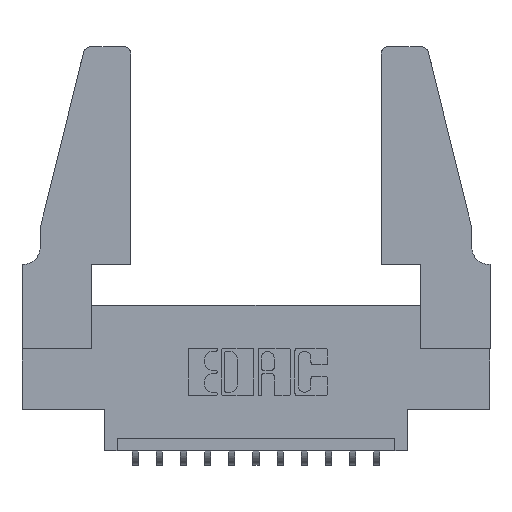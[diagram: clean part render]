
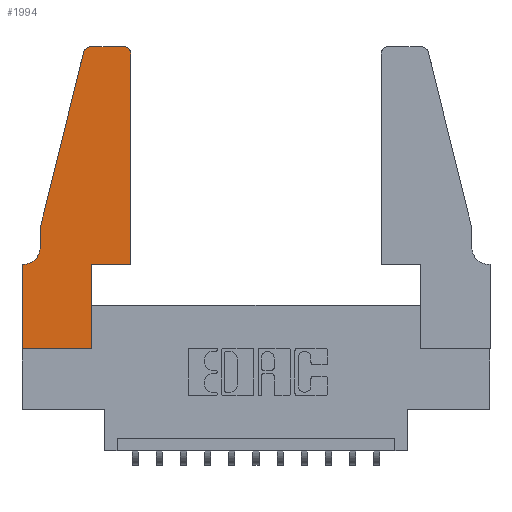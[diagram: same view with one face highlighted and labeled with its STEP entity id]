
A CAD part, top view. The second image highlights one B-rep face of the part: STEP entity #1994.
In plain terms, the highlighted planar face has unit normal (0, 0, 1).
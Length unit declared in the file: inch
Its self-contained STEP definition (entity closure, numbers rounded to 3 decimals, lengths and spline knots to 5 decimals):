
#477 = CIRCLE ( 'NONE', #2030, 0.03 ) ;
#761 = EDGE_CURVE ( 'NONE', #6258, #11032, #4310, .T. ) ;
#1099 = CARTESIAN_POINT ( 'NONE',  ( 0., 0.35, 0.37 ) ) ;
#1384 = DIRECTION ( 'NONE',  ( -1., 0., 0. ) ) ;
#1393 = VERTEX_POINT ( 'NONE', #7860 ) ;
#1628 = ORIENTED_EDGE ( 'NONE', *, *, #12560, .T. ) ;
#1816 = EDGE_CURVE ( 'NONE', #11215, #7430, #12489, .T. ) ;
#1901 = CARTESIAN_POINT ( 'NONE',  ( 0.4505, 0.35, 0.37 ) ) ;
#1978 = CARTESIAN_POINT ( 'NONE',  ( 0., 0.35, 0.37 ) ) ;
#1994 = ADVANCED_FACE ( 'NONE', ( #3218 ), #10353, .T. ) ;
#2030 = AXIS2_PLACEMENT_3D ( 'NONE', #9277, #3064, #12855 ) ;
#2187 = DIRECTION ( 'NONE',  ( 0., 0., 1. ) ) ;
#2191 = LINE ( 'NONE', #6546, #3615 ) ;
#2400 = CIRCLE ( 'NONE', #6021, 0.03 ) ;
#2414 = DIRECTION ( 'NONE',  ( 1., 0., 0. ) ) ;
#2422 = CARTESIAN_POINT ( 'NONE',  ( 0.0755, 0.42, 0.37 ) ) ;
#2580 = AXIS2_PLACEMENT_3D ( 'NONE', #4893, #10802, #13399 ) ;
#2738 = VERTEX_POINT ( 'NONE', #6799 ) ;
#2871 = CARTESIAN_POINT ( 'NONE',  ( 0.4205, 1.22, 0.37 ) ) ;
#3064 = DIRECTION ( 'NONE',  ( 0., 0., 1. ) ) ;
#3211 = VECTOR ( 'NONE', #9540, 39.37008 ) ;
#3218 = FACE_OUTER_BOUND ( 'NONE', #13090, .T. ) ;
#3220 = CARTESIAN_POINT ( 'NONE',  ( 0.284, 1.25, 0.37 ) ) ;
#3224 = VERTEX_POINT ( 'NONE', #11091 ) ;
#3413 = CARTESIAN_POINT ( 'NONE',  ( 0.0055, 0.35, 0.37 ) ) ;
#3503 = CIRCLE ( 'NONE', #2580, 0.07 ) ;
#3611 = CARTESIAN_POINT ( 'NONE',  ( 0.2865, 0.35, 0.37 ) ) ;
#3615 = VECTOR ( 'NONE', #13312, 39.37008 ) ;
#3665 = DIRECTION ( 'NONE',  ( 0., 1., 0. ) ) ;
#3710 = LINE ( 'NONE', #7285, #3211 ) ;
#3768 = EDGE_CURVE ( 'NONE', #5667, #11215, #3503, .T. ) ;
#3890 = ORIENTED_EDGE ( 'NONE', *, *, #11696, .T. ) ;
#4013 = CARTESIAN_POINT ( 'NONE',  ( 0.4505, 0.35, 0.37 ) ) ;
#4136 = CARTESIAN_POINT ( 'NONE',  ( 0.4205, 1.25, 0.37 ) ) ;
#4310 = LINE ( 'NONE', #1901, #13050 ) ;
#4850 = ORIENTED_EDGE ( 'NONE', *, *, #7431, .T. ) ;
#4851 = LINE ( 'NONE', #3611, #7729 ) ;
#4888 = ORIENTED_EDGE ( 'NONE', *, *, #5160, .T. ) ;
#4893 = CARTESIAN_POINT ( 'NONE',  ( 0.0055, 0.42, 0.37 ) ) ;
#5160 = EDGE_CURVE ( 'NONE', #7430, #11505, #2191, .T. ) ;
#5239 = ORIENTED_EDGE ( 'NONE', *, *, #7018, .T. ) ;
#5482 = ORIENTED_EDGE ( 'NONE', *, *, #761, .T. ) ;
#5501 = LINE ( 'NONE', #4013, #9078 ) ;
#5667 = VERTEX_POINT ( 'NONE', #2422 ) ;
#5742 = LINE ( 'NONE', #12825, #9144 ) ;
#5784 = VERTEX_POINT ( 'NONE', #3220 ) ;
#6021 = AXIS2_PLACEMENT_3D ( 'NONE', #2871, #2187, #11191 ) ;
#6158 = ORIENTED_EDGE ( 'NONE', *, *, #12917, .T. ) ;
#6258 = VERTEX_POINT ( 'NONE', #7651 ) ;
#6502 = CARTESIAN_POINT ( 'NONE',  ( 0.0755, 0.35, 0.37 ) ) ;
#6546 = CARTESIAN_POINT ( 'NONE',  ( 0., 0., 0.37 ) ) ;
#6591 = DIRECTION ( 'NONE',  ( -1., 0., 0. ) ) ;
#6799 = CARTESIAN_POINT ( 'NONE',  ( 0.2865, 0., 0.37 ) ) ;
#6992 = DIRECTION ( 'NONE',  ( -0.239, -0.971, 0. ) ) ;
#7018 = EDGE_CURVE ( 'NONE', #5784, #1393, #477, .T. ) ;
#7130 = CARTESIAN_POINT ( 'NONE',  ( 0.2605, 1.25, 0.37 ) ) ;
#7261 = ORIENTED_EDGE ( 'NONE', *, *, #14366, .T. ) ;
#7280 = EDGE_CURVE ( 'NONE', #3224, #6258, #5501, .T. ) ;
#7285 = CARTESIAN_POINT ( 'NONE',  ( 0., 0., 0.37 ) ) ;
#7430 = VERTEX_POINT ( 'NONE', #1978 ) ;
#7431 = EDGE_CURVE ( 'NONE', #11505, #2738, #3710, .T. ) ;
#7651 = CARTESIAN_POINT ( 'NONE',  ( 0.4505, 0.35, 0.37 ) ) ;
#7699 = AXIS2_PLACEMENT_3D ( 'NONE', #1099, #11514, #2414 ) ;
#7729 = VECTOR ( 'NONE', #3665, 39.37008 ) ;
#7860 = CARTESIAN_POINT ( 'NONE',  ( 0.25487, 1.22718, 0.37 ) ) ;
#7876 = LINE ( 'NONE', #7130, #14327 ) ;
#9032 = ORIENTED_EDGE ( 'NONE', *, *, #1816, .T. ) ;
#9078 = VECTOR ( 'NONE', #13237, 39.37008 ) ;
#9144 = VECTOR ( 'NONE', #6992, 39.37008 ) ;
#9277 = CARTESIAN_POINT ( 'NONE',  ( 0.284, 1.22, 0.37 ) ) ;
#9319 = VECTOR ( 'NONE', #14143, 39.37008 ) ;
#9540 = DIRECTION ( 'NONE',  ( 1., 0., 0. ) ) ;
#9585 = CARTESIAN_POINT ( 'NONE',  ( 0., 0., 0.37 ) ) ;
#10069 = CARTESIAN_POINT ( 'NONE',  ( 0.0755, 0.5, 0.37 ) ) ;
#10111 = ORIENTED_EDGE ( 'NONE', *, *, #7280, .T. ) ;
#10353 = PLANE ( 'NONE',  #7699 ) ;
#10649 = CARTESIAN_POINT ( 'NONE',  ( 0.0755, 0.5, 0.37 ) ) ;
#10802 = DIRECTION ( 'NONE',  ( 0., 0., -1. ) ) ;
#11032 = VERTEX_POINT ( 'NONE', #14418 ) ;
#11091 = CARTESIAN_POINT ( 'NONE',  ( 0.2865, 0.35, 0.37 ) ) ;
#11191 = DIRECTION ( 'NONE',  ( 1., 0., 0. ) ) ;
#11215 = VERTEX_POINT ( 'NONE', #3413 ) ;
#11414 = ORIENTED_EDGE ( 'NONE', *, *, #14059, .T. ) ;
#11505 = VERTEX_POINT ( 'NONE', #9585 ) ;
#11514 = DIRECTION ( 'NONE',  ( 0., 0., 1. ) ) ;
#11696 = EDGE_CURVE ( 'NONE', #13260, #5784, #7876, .T. ) ;
#11845 = LINE ( 'NONE', #10649, #9319 ) ;
#12100 = DIRECTION ( 'NONE',  ( 0., 1., 0. ) ) ;
#12489 = LINE ( 'NONE', #6502, #12666 ) ;
#12560 = EDGE_CURVE ( 'NONE', #11032, #13260, #2400, .T. ) ;
#12666 = VECTOR ( 'NONE', #6591, 39.37008 ) ;
#12825 = CARTESIAN_POINT ( 'NONE',  ( 0.0755, 0.5, 0.37 ) ) ;
#12855 = DIRECTION ( 'NONE',  ( 1., 0., 0. ) ) ;
#12917 = EDGE_CURVE ( 'NONE', #2738, #3224, #4851, .T. ) ;
#13050 = VECTOR ( 'NONE', #12100, 39.37008 ) ;
#13090 = EDGE_LOOP ( 'NONE', ( #3890, #5239, #7261, #11414, #13294, #9032, #4888, #4850, #6158, #10111, #5482, #1628 ) ) ;
#13237 = DIRECTION ( 'NONE',  ( 1., 0., 0. ) ) ;
#13260 = VERTEX_POINT ( 'NONE', #4136 ) ;
#13294 = ORIENTED_EDGE ( 'NONE', *, *, #3768, .T. ) ;
#13312 = DIRECTION ( 'NONE',  ( 0., -1., 0. ) ) ;
#13399 = DIRECTION ( 'NONE',  ( -1., 0., 0. ) ) ;
#14059 = EDGE_CURVE ( 'NONE', #14326, #5667, #11845, .T. ) ;
#14143 = DIRECTION ( 'NONE',  ( 0., -1., 0. ) ) ;
#14326 = VERTEX_POINT ( 'NONE', #10069 ) ;
#14327 = VECTOR ( 'NONE', #1384, 39.37008 ) ;
#14366 = EDGE_CURVE ( 'NONE', #1393, #14326, #5742, .T. ) ;
#14418 = CARTESIAN_POINT ( 'NONE',  ( 0.4505, 1.22, 0.37 ) ) ;
